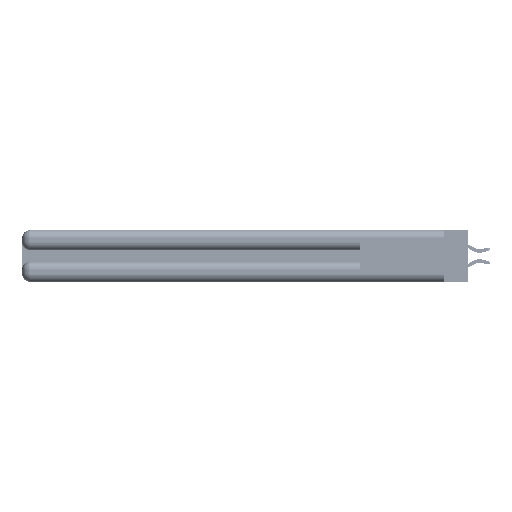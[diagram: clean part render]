
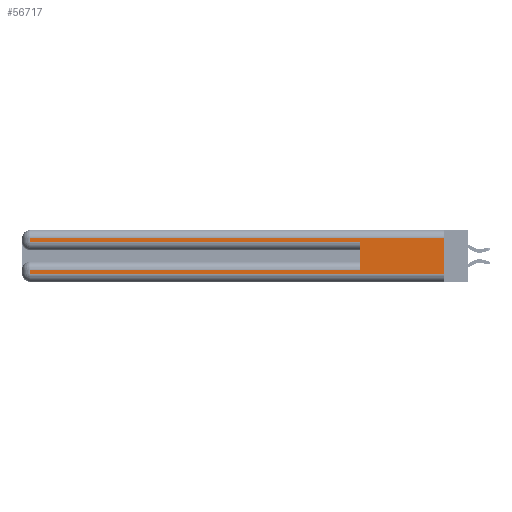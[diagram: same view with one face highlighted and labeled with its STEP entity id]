
A CAD part, left-side view. The second image highlights one B-rep face of the part: STEP entity #56717.
In plain terms, the highlighted planar face has unit normal (-1, 0, 0).
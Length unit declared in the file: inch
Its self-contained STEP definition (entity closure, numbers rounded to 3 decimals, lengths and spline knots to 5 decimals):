
#12 = CARTESIAN_POINT ( 'NONE',  ( 0., 0.6, 0.085 ) ) ;
#1443 = DIRECTION ( 'NONE',  ( 0., 1., 0. ) ) ;
#1556 = VECTOR ( 'NONE', #12164, 39.37008 ) ;
#3710 = LINE ( 'NONE', #38995, #1556 ) ;
#3822 = CARTESIAN_POINT ( 'NONE',  ( 0., 2.94, 0.285 ) ) ;
#4817 = CARTESIAN_POINT ( 'NONE',  ( 0., 0., 0.06 ) ) ;
#7932 = ORIENTED_EDGE ( 'NONE', *, *, #29441, .F. ) ;
#8620 = DIRECTION ( 'NONE',  ( 0., 0., -1. ) ) ;
#8900 = ORIENTED_EDGE ( 'NONE', *, *, #46520, .T. ) ;
#9882 = CARTESIAN_POINT ( 'NONE',  ( 0., 2.94, 0.06 ) ) ;
#11563 = LINE ( 'NONE', #24174, #45879 ) ;
#12164 = DIRECTION ( 'NONE',  ( 0., -1., 0. ) ) ;
#13700 = AXIS2_PLACEMENT_3D ( 'NONE', #39964, #48985, #8620 ) ;
#14836 = ORIENTED_EDGE ( 'NONE', *, *, #18325, .T. ) ;
#16604 = EDGE_CURVE ( 'NONE', #51698, #38978, #57863, .T. ) ;
#16625 = CARTESIAN_POINT ( 'NONE',  ( 0., 0., 0.31 ) ) ;
#18325 = EDGE_CURVE ( 'NONE', #43110, #25353, #3710, .T. ) ;
#23114 = DIRECTION ( 'NONE',  ( 0., -1., 0. ) ) ;
#24174 = CARTESIAN_POINT ( 'NONE',  ( 0., 0., 0.085 ) ) ;
#24686 = CARTESIAN_POINT ( 'NONE',  ( 0., 2.94, 0.37 ) ) ;
#25353 = VERTEX_POINT ( 'NONE', #4817 ) ;
#25438 = EDGE_CURVE ( 'NONE', #36694, #38978, #30741, .T. ) ;
#26324 = EDGE_CURVE ( 'NONE', #29399, #48648, #33433, .T. ) ;
#27222 = DIRECTION ( 'NONE',  ( 0., 0., -1. ) ) ;
#27384 = ORIENTED_EDGE ( 'NONE', *, *, #16604, .T. ) ;
#29111 = VECTOR ( 'NONE', #23114, 39.37008 ) ;
#29399 = VERTEX_POINT ( 'NONE', #16625 ) ;
#29441 = EDGE_CURVE ( 'NONE', #29399, #25353, #57729, .T. ) ;
#30101 = DIRECTION ( 'NONE',  ( 0., 0., -1. ) ) ;
#30174 = LINE ( 'NONE', #54076, #47734 ) ;
#30741 = LINE ( 'NONE', #32792, #48290 ) ;
#32792 = CARTESIAN_POINT ( 'NONE',  ( 0., 0.6, 0.145 ) ) ;
#33433 = LINE ( 'NONE', #51762, #57979 ) ;
#34564 = FACE_OUTER_BOUND ( 'NONE', #47853, .T. ) ;
#34975 = ORIENTED_EDGE ( 'NONE', *, *, #25438, .F. ) ;
#35264 = PLANE ( 'NONE',  #13700 ) ;
#36694 = VERTEX_POINT ( 'NONE', #12 ) ;
#36831 = ORIENTED_EDGE ( 'NONE', *, *, #42156, .T. ) ;
#38760 = VECTOR ( 'NONE', #30101, 39.37008 ) ;
#38978 = VERTEX_POINT ( 'NONE', #53354 ) ;
#38995 = CARTESIAN_POINT ( 'NONE',  ( 0., 0., 0.06 ) ) ;
#39964 = CARTESIAN_POINT ( 'NONE',  ( 0., 0., 0.37 ) ) ;
#41826 = DIRECTION ( 'NONE',  ( 0., 0., 1. ) ) ;
#42117 = DIRECTION ( 'NONE',  ( 0., 0., -1. ) ) ;
#42156 = EDGE_CURVE ( 'NONE', #36694, #45144, #11563, .T. ) ;
#43110 = VERTEX_POINT ( 'NONE', #9882 ) ;
#44223 = CARTESIAN_POINT ( 'NONE',  ( 0., 0., 0.37 ) ) ;
#45144 = VERTEX_POINT ( 'NONE', #50198 ) ;
#45335 = ORIENTED_EDGE ( 'NONE', *, *, #26324, .T. ) ;
#45750 = EDGE_CURVE ( 'NONE', #45144, #43110, #49931, .T. ) ;
#45879 = VECTOR ( 'NONE', #1443, 39.37008 ) ;
#46520 = EDGE_CURVE ( 'NONE', #48648, #51698, #30174, .T. ) ;
#46984 = CARTESIAN_POINT ( 'NONE',  ( 0., 2.94, 0.31 ) ) ;
#47734 = VECTOR ( 'NONE', #27222, 39.37008 ) ;
#47853 = EDGE_LOOP ( 'NONE', ( #7932, #45335, #8900, #27384, #34975, #36831, #51434, #14836 ) ) ;
#48290 = VECTOR ( 'NONE', #41826, 39.37008 ) ;
#48648 = VERTEX_POINT ( 'NONE', #46984 ) ;
#48985 = DIRECTION ( 'NONE',  ( 1., 0., 0. ) ) ;
#49577 = CARTESIAN_POINT ( 'NONE',  ( 0., 0., 0.285 ) ) ;
#49931 = LINE ( 'NONE', #24686, #52755 ) ;
#50198 = CARTESIAN_POINT ( 'NONE',  ( 0., 2.94, 0.085 ) ) ;
#51434 = ORIENTED_EDGE ( 'NONE', *, *, #45750, .T. ) ;
#51698 = VERTEX_POINT ( 'NONE', #3822 ) ;
#51762 = CARTESIAN_POINT ( 'NONE',  ( 0., 0., 0.31 ) ) ;
#51951 = DIRECTION ( 'NONE',  ( 0., 1., 0. ) ) ;
#52755 = VECTOR ( 'NONE', #42117, 39.37008 ) ;
#53354 = CARTESIAN_POINT ( 'NONE',  ( 0., 0.6, 0.285 ) ) ;
#54076 = CARTESIAN_POINT ( 'NONE',  ( 0., 2.94, 0.37 ) ) ;
#56717 = ADVANCED_FACE ( 'NONE', ( #34564 ), #35264, .F. ) ;
#57729 = LINE ( 'NONE', #44223, #38760 ) ;
#57863 = LINE ( 'NONE', #49577, #29111 ) ;
#57979 = VECTOR ( 'NONE', #51951, 39.37008 ) ;
